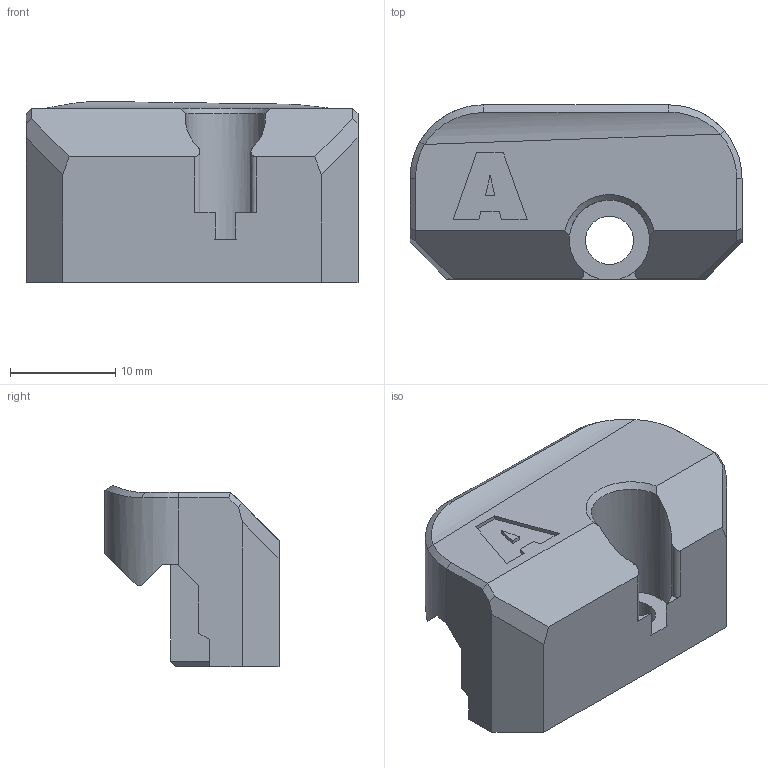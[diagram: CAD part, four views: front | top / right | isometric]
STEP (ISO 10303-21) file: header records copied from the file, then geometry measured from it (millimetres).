
FILE_DESCRIPTION (( 'STEP AP214' ), '1' );
FILE_NAME ('Chassis - Key.STEP', '2022-02-04T02:39:15', ( '' ), ( '' ), 'SwSTEP 2.0', 'SolidWorks 2020', '' );
FILE_SCHEMA (( 'AUTOMOTIVE_DESIGN' ));
Length unit declared in the file: inch
Products named in the file (1): Chassis - Key
Bounding box: 31.5 x 16.51 x 17.17 mm (x, y, z)
Volume: 4904.9 mm3; surface area: 2458.7 mm2
Topology: 1 solids, 1 shells, 71 faces, 191 edges, 124 vertices
Faces by surface type: plane 52, cylinder 11, bspline 5, cone 3
Entity records: 2656 total; most frequent: CARTESIAN_POINT 898, ORIENTED_EDGE 382, DIRECTION 318, EDGE_CURVE 191, LINE 140, VECTOR 140, VERTEX_POINT 124, AXIS2_PLACEMENT_3D 89
